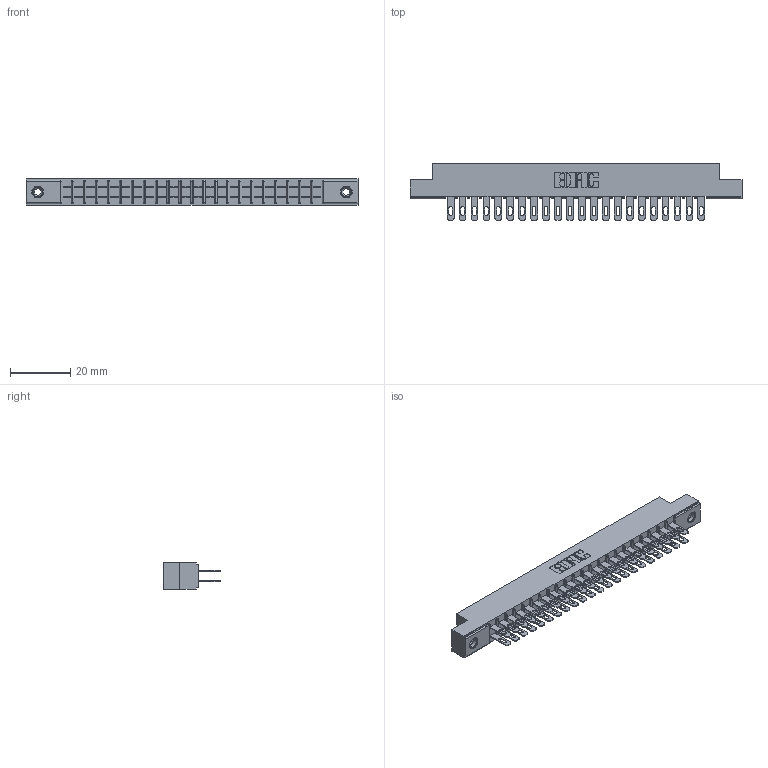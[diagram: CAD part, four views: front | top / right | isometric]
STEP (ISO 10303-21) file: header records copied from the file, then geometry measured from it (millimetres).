
FILE_DESCRIPTION (( 'STEP AP203' ), '1' );
FILE_NAME ('305-044-500-208.STEP', '2019-09-09T19:48:15', ( '' ), ( '' ), 'SwSTEP 2.0', 'SolidWorks 2016', '' );
FILE_SCHEMA (( 'CONFIG_CONTROL_DESIGN' ));
Length unit declared in the file: inch
Products named in the file (4): 305-290-001_500; 345-250-001_345-250-003-102; 305 Part_.156 Dia; 305-044-500-208
Assembly tree (47 placements, depth 2):
  305-044-500-208
    305 Part_.156 Dia
    305-290-001_500  x44
    345-250-001_345-250-003-102  x2
Bounding box: 110.19 x 18.85 x 8.71 mm (x, y, z)
Volume: 7035.8 mm3; surface area: 14095.3 mm2
Topology: 47 solids, 47 shells, 2376 faces, 6766 edges, 4384 vertices
Faces by surface type: plane 1332, cylinder 940, sphere 88, cone 12, torus 4
Entity records: 27462 total; most frequent: CARTESIAN_POINT 4527, ORIENTED_EDGE 4484, DIRECTION 4408, EDGE_CURVE 2242, LINE 1786, VECTOR 1786, VERTEX_POINT 1430, AXIS2_PLACEMENT_3D 1311
